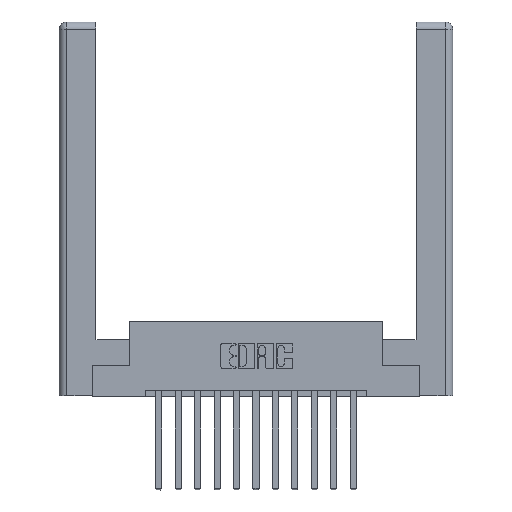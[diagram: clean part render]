
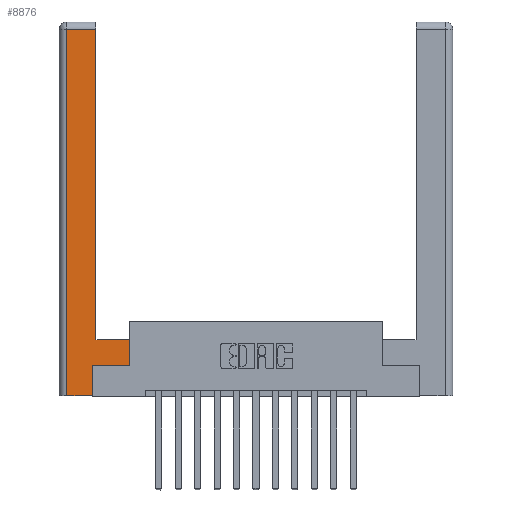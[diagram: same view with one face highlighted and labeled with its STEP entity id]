
A CAD part, top view. The second image highlights one B-rep face of the part: STEP entity #8876.
In plain terms, the highlighted planar face has unit normal (0, 0, 1).
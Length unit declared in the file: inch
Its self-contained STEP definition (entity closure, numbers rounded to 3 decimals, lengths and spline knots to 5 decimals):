
#104 = DIRECTION ( 'NONE',  ( -1., 0., 0. ) ) ;
#261 = VERTEX_POINT ( 'NONE', #13357 ) ;
#903 = CARTESIAN_POINT ( 'NONE',  ( 0.295, 0.45, 0. ) ) ;
#1248 = VECTOR ( 'NONE', #4370, 39.37008 ) ;
#1639 = CARTESIAN_POINT ( 'NONE',  ( 0.0615, 0., 0. ) ) ;
#1696 = EDGE_CURVE ( 'NONE', #2511, #261, #8345, .T. ) ;
#2300 = EDGE_CURVE ( 'NONE', #5747, #3606, #5468, .T. ) ;
#2343 = LINE ( 'NONE', #1639, #14235 ) ;
#2511 = VERTEX_POINT ( 'NONE', #8863 ) ;
#2574 = EDGE_CURVE ( 'NONE', #14208, #5747, #10810, .T. ) ;
#2774 = DIRECTION ( 'NONE',  ( 0., -1., 0. ) ) ;
#3030 = EDGE_CURVE ( 'NONE', #10901, #14208, #8821, .T. ) ;
#3221 = DIRECTION ( 'NONE',  ( 1., 0., 0. ) ) ;
#3329 = EDGE_CURVE ( 'NONE', #3606, #2511, #14062, .T. ) ;
#3535 = CARTESIAN_POINT ( 'NONE',  ( 0., 0., 0. ) ) ;
#3606 = VERTEX_POINT ( 'NONE', #4910 ) ;
#3885 = FACE_OUTER_BOUND ( 'NONE', #14215, .T. ) ;
#4044 = LINE ( 'NONE', #14730, #14518 ) ;
#4370 = DIRECTION ( 'NONE',  ( 0., 1., 0. ) ) ;
#4387 = ORIENTED_EDGE ( 'NONE', *, *, #7375, .T. ) ;
#4496 = EDGE_CURVE ( 'NONE', #9572, #9048, #14948, .T. ) ;
#4910 = CARTESIAN_POINT ( 'NONE',  ( 0.565, 0.245, 0. ) ) ;
#5185 = CARTESIAN_POINT ( 'NONE',  ( 0.265, 0., 0. ) ) ;
#5431 = DIRECTION ( 'NONE',  ( -1., 0., 0. ) ) ;
#5468 = LINE ( 'NONE', #6598, #5559 ) ;
#5559 = VECTOR ( 'NONE', #3221, 39.37008 ) ;
#5747 = VERTEX_POINT ( 'NONE', #14764 ) ;
#5783 = ORIENTED_EDGE ( 'NONE', *, *, #2300, .T. ) ;
#6136 = DIRECTION ( 'NONE',  ( -1., 0., 0. ) ) ;
#6598 = CARTESIAN_POINT ( 'NONE',  ( 0.565, 0.245, 0. ) ) ;
#6901 = CARTESIAN_POINT ( 'NONE',  ( 0.0615, 0., 0. ) ) ;
#7064 = DIRECTION ( 'NONE',  ( 0., 0., -1. ) ) ;
#7375 = EDGE_CURVE ( 'NONE', #261, #9572, #4044, .T. ) ;
#7484 = DIRECTION ( 'NONE',  ( 0., 1., 0. ) ) ;
#7901 = VECTOR ( 'NONE', #6136, 39.37008 ) ;
#8223 = ORIENTED_EDGE ( 'NONE', *, *, #3329, .T. ) ;
#8345 = LINE ( 'NONE', #903, #12334 ) ;
#8626 = ORIENTED_EDGE ( 'NONE', *, *, #3030, .T. ) ;
#8821 = LINE ( 'NONE', #11663, #14628 ) ;
#8863 = CARTESIAN_POINT ( 'NONE',  ( 0.565, 0.45, 0. ) ) ;
#8876 = ADVANCED_FACE ( 'NONE', ( #3885 ), #12025, .F. ) ;
#9048 = VERTEX_POINT ( 'NONE', #12281 ) ;
#9225 = DIRECTION ( 'NONE',  ( 1., 0., 0. ) ) ;
#9572 = VERTEX_POINT ( 'NONE', #9688 ) ;
#9688 = CARTESIAN_POINT ( 'NONE',  ( 0.295, 2.94, 0. ) ) ;
#9692 = CARTESIAN_POINT ( 'NONE',  ( 0.0615, 2.94, 0. ) ) ;
#10810 = LINE ( 'NONE', #12366, #1248 ) ;
#10901 = VERTEX_POINT ( 'NONE', #6901 ) ;
#11522 = VECTOR ( 'NONE', #7484, 39.37008 ) ;
#11663 = CARTESIAN_POINT ( 'NONE',  ( 0.265, 0., 0. ) ) ;
#12025 = PLANE ( 'NONE',  #14722 ) ;
#12281 = CARTESIAN_POINT ( 'NONE',  ( 0.0615, 2.94, 0. ) ) ;
#12334 = VECTOR ( 'NONE', #5431, 39.37008 ) ;
#12366 = CARTESIAN_POINT ( 'NONE',  ( 0.265, 0.245, 0. ) ) ;
#12636 = EDGE_CURVE ( 'NONE', #9048, #10901, #2343, .T. ) ;
#12759 = ORIENTED_EDGE ( 'NONE', *, *, #12636, .T. ) ;
#13343 = DIRECTION ( 'NONE',  ( 0., 1., 0. ) ) ;
#13357 = CARTESIAN_POINT ( 'NONE',  ( 0.295, 0.45, 0. ) ) ;
#13709 = ORIENTED_EDGE ( 'NONE', *, *, #2574, .T. ) ;
#13759 = ORIENTED_EDGE ( 'NONE', *, *, #4496, .T. ) ;
#14062 = LINE ( 'NONE', #14394, #11522 ) ;
#14208 = VERTEX_POINT ( 'NONE', #5185 ) ;
#14215 = EDGE_LOOP ( 'NONE', ( #4387, #13759, #12759, #8626, #13709, #5783, #8223, #14558 ) ) ;
#14235 = VECTOR ( 'NONE', #2774, 39.37008 ) ;
#14394 = CARTESIAN_POINT ( 'NONE',  ( 0.565, 0.45, 0. ) ) ;
#14518 = VECTOR ( 'NONE', #13343, 39.37008 ) ;
#14558 = ORIENTED_EDGE ( 'NONE', *, *, #1696, .T. ) ;
#14628 = VECTOR ( 'NONE', #9225, 39.37008 ) ;
#14722 = AXIS2_PLACEMENT_3D ( 'NONE', #3535, #7064, #104 ) ;
#14730 = CARTESIAN_POINT ( 'NONE',  ( 0.295, 3., 0. ) ) ;
#14764 = CARTESIAN_POINT ( 'NONE',  ( 0.265, 0.245, 0. ) ) ;
#14948 = LINE ( 'NONE', #9692, #7901 ) ;
